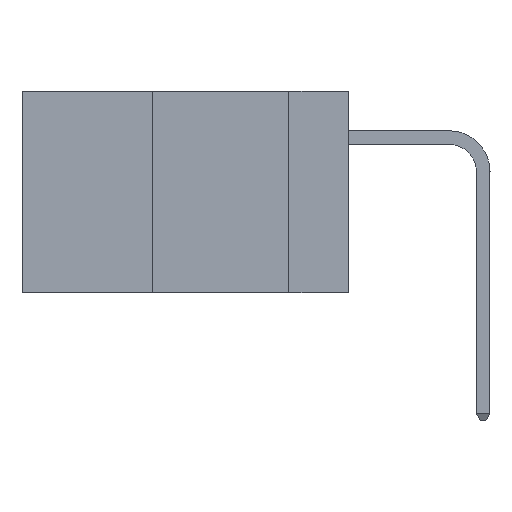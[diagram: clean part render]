
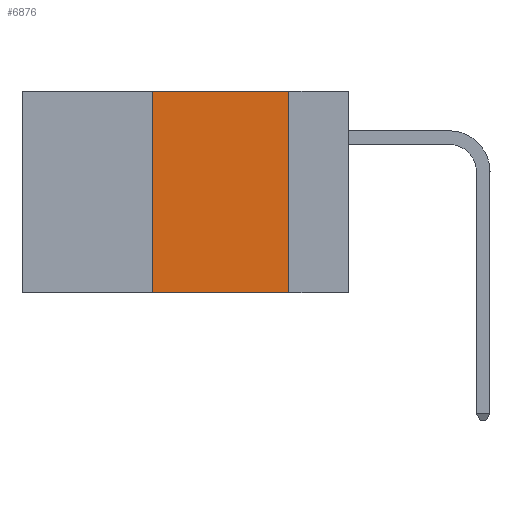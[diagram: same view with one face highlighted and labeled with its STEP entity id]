
A CAD part, left-side view. The second image highlights one B-rep face of the part: STEP entity #6876.
In plain terms, the highlighted planar face has unit normal (-1, 0, 0).
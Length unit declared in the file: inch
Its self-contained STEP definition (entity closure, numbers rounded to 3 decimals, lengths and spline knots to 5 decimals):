
#264 = DIRECTION ( 'NONE',  ( 0., -1., 0. ) ) ;
#1007 = EDGE_CURVE ( 'NONE', #13951, #6668, #12580, .T. ) ;
#1047 = FACE_OUTER_BOUND ( 'NONE', #17198, .T. ) ;
#1414 = LINE ( 'NONE', #14415, #17896 ) ;
#1748 = DIRECTION ( 'NONE',  ( 0., 0., -1. ) ) ;
#2506 = EDGE_CURVE ( 'NONE', #9855, #13951, #15565, .T. ) ;
#2540 = DIRECTION ( 'NONE',  ( 0., -1., 0. ) ) ;
#3280 = DIRECTION ( 'NONE',  ( 0., 0., -1. ) ) ;
#4664 = ORIENTED_EDGE ( 'NONE', *, *, #16173, .F. ) ;
#4826 = ORIENTED_EDGE ( 'NONE', *, *, #1007, .F. ) ;
#4886 = AXIS2_PLACEMENT_3D ( 'NONE', #15818, #10245, #1748 ) ;
#5556 = CARTESIAN_POINT ( 'NONE',  ( 0., 0.11, 0. ) ) ;
#6077 = CARTESIAN_POINT ( 'NONE',  ( 0., 0.11, 0. ) ) ;
#6668 = VERTEX_POINT ( 'NONE', #5556 ) ;
#6876 = ADVANCED_FACE ( 'NONE', ( #1047 ), #13045, .F. ) ;
#7201 = VECTOR ( 'NONE', #7909, 39.37008 ) ;
#7909 = DIRECTION ( 'NONE',  ( 0., 0., 1. ) ) ;
#8863 = CARTESIAN_POINT ( 'NONE',  ( 0., 0.11, -0.37 ) ) ;
#9855 = VERTEX_POINT ( 'NONE', #15213 ) ;
#10149 = VERTEX_POINT ( 'NONE', #8863 ) ;
#10245 = DIRECTION ( 'NONE',  ( 1., 0., 0. ) ) ;
#10506 = ORIENTED_EDGE ( 'NONE', *, *, #2506, .F. ) ;
#11406 = EDGE_CURVE ( 'NONE', #9855, #10149, #1414, .T. ) ;
#11696 = CARTESIAN_POINT ( 'NONE',  ( 0., 0.36, 0. ) ) ;
#11887 = CARTESIAN_POINT ( 'NONE',  ( 0., 0.36, 0. ) ) ;
#12129 = VECTOR ( 'NONE', #3280, 39.37008 ) ;
#12573 = LINE ( 'NONE', #6077, #12129 ) ;
#12580 = LINE ( 'NONE', #17731, #15829 ) ;
#13045 = PLANE ( 'NONE',  #4886 ) ;
#13951 = VERTEX_POINT ( 'NONE', #11696 ) ;
#14415 = CARTESIAN_POINT ( 'NONE',  ( 0., 0.6, -0.37 ) ) ;
#15213 = CARTESIAN_POINT ( 'NONE',  ( 0., 0.36, -0.37 ) ) ;
#15565 = LINE ( 'NONE', #11887, #7201 ) ;
#15652 = ORIENTED_EDGE ( 'NONE', *, *, #11406, .T. ) ;
#15818 = CARTESIAN_POINT ( 'NONE',  ( 0., 0.6, 0. ) ) ;
#15829 = VECTOR ( 'NONE', #2540, 39.37008 ) ;
#16173 = EDGE_CURVE ( 'NONE', #6668, #10149, #12573, .T. ) ;
#17198 = EDGE_LOOP ( 'NONE', ( #4664, #4826, #10506, #15652 ) ) ;
#17731 = CARTESIAN_POINT ( 'NONE',  ( 0., 0.6, 0. ) ) ;
#17896 = VECTOR ( 'NONE', #264, 39.37008 ) ;
